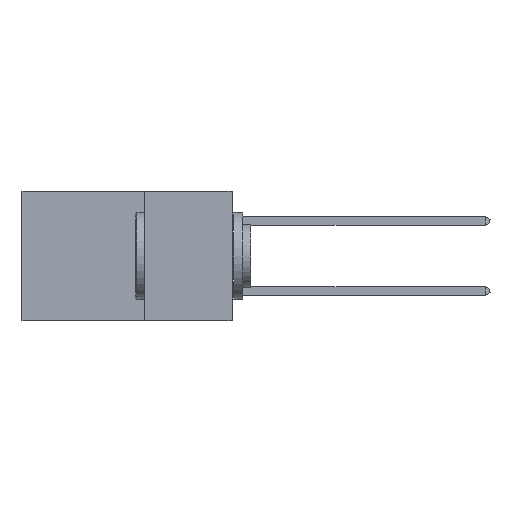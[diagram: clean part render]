
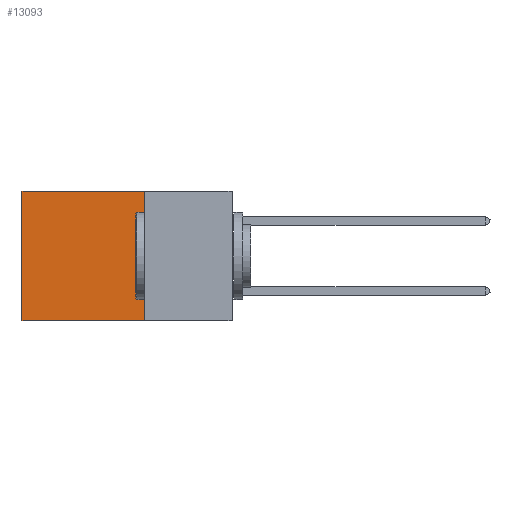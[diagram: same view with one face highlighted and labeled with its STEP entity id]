
A CAD part, left-side view. The second image highlights one B-rep face of the part: STEP entity #13093.
In plain terms, the highlighted planar face has unit normal (-1, 0, 0).
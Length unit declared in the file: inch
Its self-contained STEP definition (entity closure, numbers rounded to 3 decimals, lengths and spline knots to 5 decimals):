
#444 = FACE_OUTER_BOUND ( 'NONE', #20187, .T. ) ;
#3064 = AXIS2_PLACEMENT_3D ( 'NONE', #24828, #17760, #24686 ) ;
#3482 = PLANE ( 'NONE',  #3064 ) ;
#4001 = DIRECTION ( 'NONE',  ( 0., 0., -1. ) ) ;
#4346 = DIRECTION ( 'NONE',  ( 0., 0., -1. ) ) ;
#6342 = DIRECTION ( 'NONE',  ( 0., 1., 0. ) ) ;
#7704 = VECTOR ( 'NONE', #6342, 39.37008 ) ;
#9187 = VECTOR ( 'NONE', #4001, 39.37008 ) ;
#9571 = ORIENTED_EDGE ( 'NONE', *, *, #26573, .F. ) ;
#9586 = CARTESIAN_POINT ( 'NONE',  ( 0.2875, 0.6, 0. ) ) ;
#11377 = VERTEX_POINT ( 'NONE', #11574 ) ;
#11574 = CARTESIAN_POINT ( 'NONE',  ( 0.2875, 0.6, -0.37 ) ) ;
#11862 = CARTESIAN_POINT ( 'NONE',  ( 0.2875, 0.25, -0.37 ) ) ;
#12165 = DIRECTION ( 'NONE',  ( 0., 1., 0. ) ) ;
#12421 = VECTOR ( 'NONE', #12165, 39.37008 ) ;
#13093 = ADVANCED_FACE ( 'NONE', ( #444 ), #3482, .F. ) ;
#13291 = VECTOR ( 'NONE', #4346, 39.37008 ) ;
#13915 = EDGE_CURVE ( 'NONE', #45250, #11377, #36321, .T. ) ;
#16948 = ORIENTED_EDGE ( 'NONE', *, *, #21573, .T. ) ;
#17760 = DIRECTION ( 'NONE',  ( 1., 0., 0. ) ) ;
#20187 = EDGE_LOOP ( 'NONE', ( #16948, #34265, #9571, #22741 ) ) ;
#21573 = EDGE_CURVE ( 'NONE', #39108, #11377, #31654, .T. ) ;
#22741 = ORIENTED_EDGE ( 'NONE', *, *, #35082, .T. ) ;
#24686 = DIRECTION ( 'NONE',  ( 0., 0., -1. ) ) ;
#24828 = CARTESIAN_POINT ( 'NONE',  ( 0.2875, 0.25, 0. ) ) ;
#26573 = EDGE_CURVE ( 'NONE', #27769, #45250, #34013, .T. ) ;
#27586 = LINE ( 'NONE', #41170, #12421 ) ;
#27769 = VERTEX_POINT ( 'NONE', #30943 ) ;
#29127 = CARTESIAN_POINT ( 'NONE',  ( 0.2875, 0.25, 0. ) ) ;
#30943 = CARTESIAN_POINT ( 'NONE',  ( 0.2875, 0.25, 0. ) ) ;
#31654 = LINE ( 'NONE', #43334, #9187 ) ;
#34013 = LINE ( 'NONE', #29127, #13291 ) ;
#34265 = ORIENTED_EDGE ( 'NONE', *, *, #13915, .F. ) ;
#35082 = EDGE_CURVE ( 'NONE', #27769, #39108, #27586, .T. ) ;
#36321 = LINE ( 'NONE', #45852, #7704 ) ;
#39108 = VERTEX_POINT ( 'NONE', #9586 ) ;
#41170 = CARTESIAN_POINT ( 'NONE',  ( 0.2875, 0.25, 0. ) ) ;
#43334 = CARTESIAN_POINT ( 'NONE',  ( 0.2875, 0.6, 0. ) ) ;
#45250 = VERTEX_POINT ( 'NONE', #11862 ) ;
#45852 = CARTESIAN_POINT ( 'NONE',  ( 0.2875, 0.25, -0.37 ) ) ;
